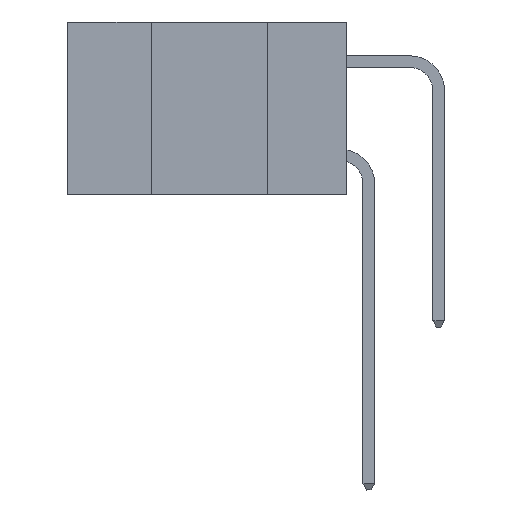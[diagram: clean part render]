
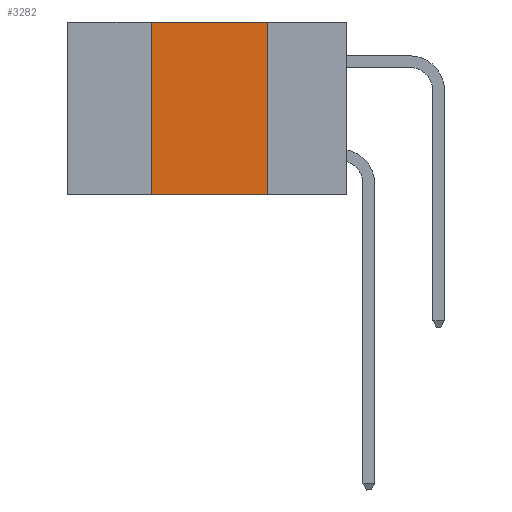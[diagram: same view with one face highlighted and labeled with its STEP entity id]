
A CAD part, left-side view. The second image highlights one B-rep face of the part: STEP entity #3282.
In plain terms, the highlighted planar face has unit normal (-1, 0, 0).
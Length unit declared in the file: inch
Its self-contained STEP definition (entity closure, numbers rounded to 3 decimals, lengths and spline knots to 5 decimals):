
#193 = EDGE_CURVE ( 'NONE', #25641, #9264, #4401, .T. ) ;
#1872 = VECTOR ( 'NONE', #9870, 39.37008 ) ;
#2106 = ORIENTED_EDGE ( 'NONE', *, *, #20123, .T. ) ;
#2617 = DIRECTION ( 'NONE',  ( 0., 0., -1. ) ) ;
#3282 = ADVANCED_FACE ( 'NONE', ( #24714 ), #24123, .F. ) ;
#4401 = LINE ( 'NONE', #12217, #1872 ) ;
#5421 = CARTESIAN_POINT ( 'NONE',  ( 0., 0.6, 0. ) ) ;
#5728 = CARTESIAN_POINT ( 'NONE',  ( 0., 0.17, 0. ) ) ;
#8230 = CARTESIAN_POINT ( 'NONE',  ( 0., 0.42, 0. ) ) ;
#8417 = ORIENTED_EDGE ( 'NONE', *, *, #193, .F. ) ;
#9264 = VERTEX_POINT ( 'NONE', #5728 ) ;
#9579 = DIRECTION ( 'NONE',  ( 0., 0., 1. ) ) ;
#9637 = CARTESIAN_POINT ( 'NONE',  ( 0., 0.42, -0.37 ) ) ;
#9870 = DIRECTION ( 'NONE',  ( 0., -1., 0. ) ) ;
#10734 = DIRECTION ( 'NONE',  ( 1., 0., 0. ) ) ;
#11720 = AXIS2_PLACEMENT_3D ( 'NONE', #5421, #10734, #2617 ) ;
#12217 = CARTESIAN_POINT ( 'NONE',  ( 0., 0.6, 0. ) ) ;
#14213 = VERTEX_POINT ( 'NONE', #33381 ) ;
#14963 = CARTESIAN_POINT ( 'NONE',  ( 0., 0.42, 0. ) ) ;
#15884 = DIRECTION ( 'NONE',  ( 0., -1., 0. ) ) ;
#16449 = LINE ( 'NONE', #20246, #27754 ) ;
#17879 = ORIENTED_EDGE ( 'NONE', *, *, #21450, .F. ) ;
#19567 = VECTOR ( 'NONE', #15884, 39.37008 ) ;
#20123 = EDGE_CURVE ( 'NONE', #20188, #14213, #33408, .T. ) ;
#20188 = VERTEX_POINT ( 'NONE', #9637 ) ;
#20246 = CARTESIAN_POINT ( 'NONE',  ( 0., 0.17, 0. ) ) ;
#21082 = CARTESIAN_POINT ( 'NONE',  ( 0., 0.6, -0.37 ) ) ;
#21450 = EDGE_CURVE ( 'NONE', #20188, #25641, #22384, .T. ) ;
#22384 = LINE ( 'NONE', #14963, #28252 ) ;
#22999 = EDGE_CURVE ( 'NONE', #9264, #14213, #16449, .T. ) ;
#24123 = PLANE ( 'NONE',  #11720 ) ;
#24714 = FACE_OUTER_BOUND ( 'NONE', #27219, .T. ) ;
#25641 = VERTEX_POINT ( 'NONE', #8230 ) ;
#27219 = EDGE_LOOP ( 'NONE', ( #32639, #8417, #17879, #2106 ) ) ;
#27754 = VECTOR ( 'NONE', #31520, 39.37008 ) ;
#28252 = VECTOR ( 'NONE', #9579, 39.37008 ) ;
#31520 = DIRECTION ( 'NONE',  ( 0., 0., -1. ) ) ;
#32639 = ORIENTED_EDGE ( 'NONE', *, *, #22999, .F. ) ;
#33381 = CARTESIAN_POINT ( 'NONE',  ( 0., 0.17, -0.37 ) ) ;
#33408 = LINE ( 'NONE', #21082, #19567 ) ;
